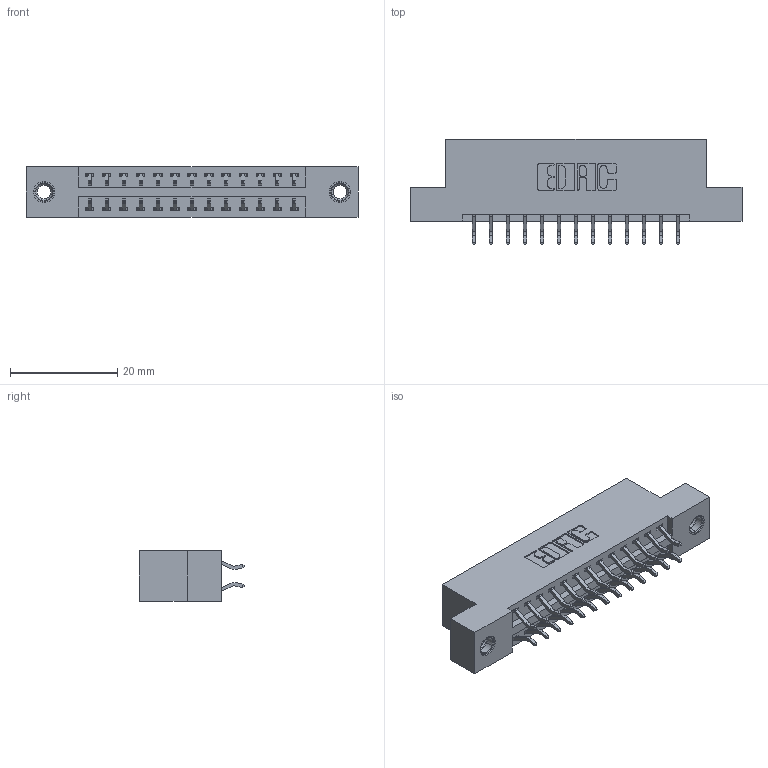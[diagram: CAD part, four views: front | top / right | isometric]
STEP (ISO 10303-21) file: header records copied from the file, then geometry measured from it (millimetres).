
FILE_DESCRIPTION (( 'STEP AP203' ), '1' );
FILE_NAME ('346-026-556-207.STEP', '2022-05-19T02:30:15', ( '' ), ( '' ), 'SwSTEP 2.0', 'SolidWorks 2020', '' );
FILE_SCHEMA (( 'CONFIG_CONTROL_DESIGN' ));
Length unit declared in the file: inch
Products named in the file (4): 345-292-001_556 Tail; 346-026-556-207; 346 Part_Flush Mounting Lugs - 0.156 Dia-TI; 345-250-001_345-250-005-103
Assembly tree (29 placements, depth 2):
  346-026-556-207
    346 Part_Flush Mounting Lugs - 0.156 Dia-TI
    345-292-001_556 Tail  x26
    345-250-001_345-250-005-103  x2
Bounding box: 61.85 x 19.57 x 9.4 mm (x, y, z)
Volume: 5791.3 mm3; surface area: 7514.3 mm2
Topology: 29 solids, 29 shells, 1690 faces, 4963 edges, 3266 vertices
Faces by surface type: plane 1122, cylinder 552, cone 12, torus 4
Entity records: 13794 total; most frequent: CARTESIAN_POINT 2311, ORIENTED_EDGE 2226, DIRECTION 2103, EDGE_CURVE 1113, LINE 901, VECTOR 901, VERTEX_POINT 736, AXIS2_PLACEMENT_3D 601
